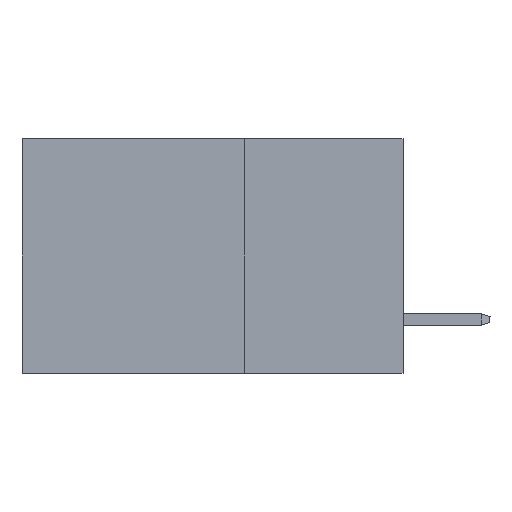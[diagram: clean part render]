
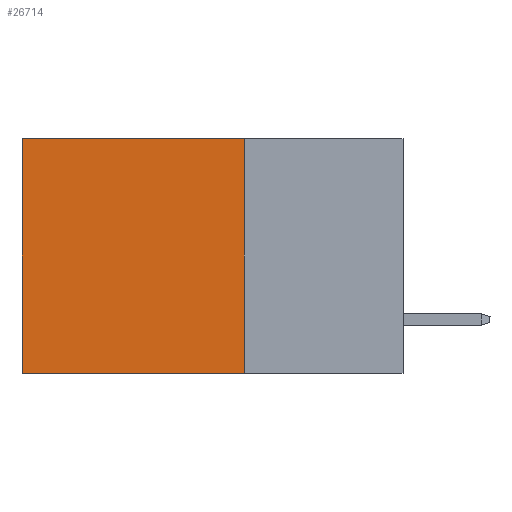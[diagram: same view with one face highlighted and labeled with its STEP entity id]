
A CAD part, left-side view. The second image highlights one B-rep face of the part: STEP entity #26714.
In plain terms, the highlighted planar face has unit normal (-1, 0, 0).
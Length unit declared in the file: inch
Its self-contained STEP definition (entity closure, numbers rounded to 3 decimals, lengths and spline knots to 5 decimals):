
#1075 = PLANE ( 'NONE',  #18913 ) ;
#2521 = CARTESIAN_POINT ( 'NONE',  ( 0.2875, 0.25, -0.37 ) ) ;
#2824 = DIRECTION ( 'NONE',  ( 0., 0., -1. ) ) ;
#2923 = LINE ( 'NONE', #28766, #21539 ) ;
#3042 = CARTESIAN_POINT ( 'NONE',  ( 0.2875, 0.6, -0.37 ) ) ;
#3522 = CARTESIAN_POINT ( 'NONE',  ( 0.2875, 0.25, 0. ) ) ;
#3650 = EDGE_LOOP ( 'NONE', ( #13245, #17395, #18904, #4400 ) ) ;
#4400 = ORIENTED_EDGE ( 'NONE', *, *, #15137, .T. ) ;
#4547 = VECTOR ( 'NONE', #21742, 39.37008 ) ;
#5835 = DIRECTION ( 'NONE',  ( 1., 0., 0. ) ) ;
#6825 = DIRECTION ( 'NONE',  ( 0., 0., -1. ) ) ;
#7688 = DIRECTION ( 'NONE',  ( 0., 1., 0. ) ) ;
#8045 = VECTOR ( 'NONE', #2824, 39.37008 ) ;
#9841 = DIRECTION ( 'NONE',  ( 0., 0., -1. ) ) ;
#10286 = FACE_OUTER_BOUND ( 'NONE', #3650, .T. ) ;
#11819 = VERTEX_POINT ( 'NONE', #29976 ) ;
#13245 = ORIENTED_EDGE ( 'NONE', *, *, #22621, .T. ) ;
#15137 = EDGE_CURVE ( 'NONE', #11819, #24783, #2923, .T. ) ;
#16504 = CARTESIAN_POINT ( 'NONE',  ( 0.2875, 0.25, 0. ) ) ;
#16643 = VERTEX_POINT ( 'NONE', #3042 ) ;
#17395 = ORIENTED_EDGE ( 'NONE', *, *, #22750, .F. ) ;
#18518 = LINE ( 'NONE', #27917, #29621 ) ;
#18816 = LINE ( 'NONE', #16504, #8045 ) ;
#18904 = ORIENTED_EDGE ( 'NONE', *, *, #21509, .F. ) ;
#18913 = AXIS2_PLACEMENT_3D ( 'NONE', #3522, #5835, #9841 ) ;
#19889 = VERTEX_POINT ( 'NONE', #23943 ) ;
#21509 = EDGE_CURVE ( 'NONE', #11819, #19889, #18816, .T. ) ;
#21539 = VECTOR ( 'NONE', #7688, 39.37008 ) ;
#21742 = DIRECTION ( 'NONE',  ( 0., 1., 0. ) ) ;
#22621 = EDGE_CURVE ( 'NONE', #24783, #16643, #18518, .T. ) ;
#22750 = EDGE_CURVE ( 'NONE', #19889, #16643, #28674, .T. ) ;
#23943 = CARTESIAN_POINT ( 'NONE',  ( 0.2875, 0.25, -0.37 ) ) ;
#24783 = VERTEX_POINT ( 'NONE', #28046 ) ;
#26714 = ADVANCED_FACE ( 'NONE', ( #10286 ), #1075, .F. ) ;
#27917 = CARTESIAN_POINT ( 'NONE',  ( 0.2875, 0.6, 0. ) ) ;
#28046 = CARTESIAN_POINT ( 'NONE',  ( 0.2875, 0.6, 0. ) ) ;
#28674 = LINE ( 'NONE', #2521, #4547 ) ;
#28766 = CARTESIAN_POINT ( 'NONE',  ( 0.2875, 0.25, 0. ) ) ;
#29621 = VECTOR ( 'NONE', #6825, 39.37008 ) ;
#29976 = CARTESIAN_POINT ( 'NONE',  ( 0.2875, 0.25, 0. ) ) ;
